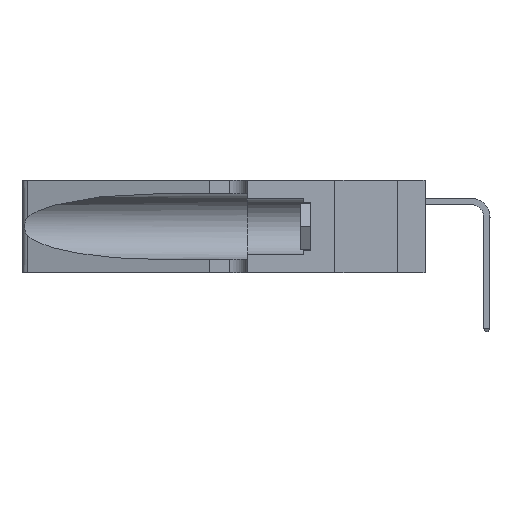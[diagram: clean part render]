
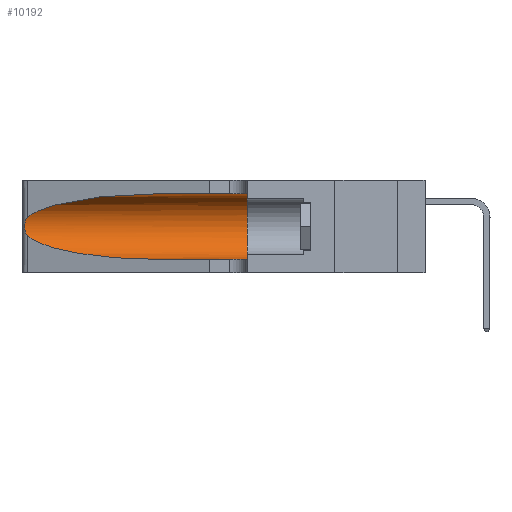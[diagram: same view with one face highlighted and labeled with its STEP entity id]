
A CAD part, left-side view. The second image highlights one B-rep face of the part: STEP entity #10192.
In plain terms, the highlighted cylindrical face has radius 3.308 mm (diameter 6.617 mm), a partial arc.
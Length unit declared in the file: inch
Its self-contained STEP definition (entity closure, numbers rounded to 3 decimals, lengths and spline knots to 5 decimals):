
#123 = CARTESIAN_POINT ( 'NONE',  ( 0.1305, 0.72297, 0.31525 ) ) ;
#985 = EDGE_LOOP ( 'NONE', ( #15493, #10895, #1255, #1177, #18945, #2947 ) ) ;
#1099 = FACE_OUTER_BOUND ( 'NONE', #985, .T. ) ;
#1177 = ORIENTED_EDGE ( 'NONE', *, *, #17334, .T. ) ;
#1226 = CARTESIAN_POINT ( 'NONE',  ( 0.1305, 0.35, 0.185 ) ) ;
#1255 = ORIENTED_EDGE ( 'NONE', *, *, #4249, .T. ) ;
#1370 = CARTESIAN_POINT ( 'NONE',  ( 0.26018, 1.23835, 0.19895 ) ) ;
#1497 = EDGE_CURVE ( 'NONE', #17183, #18191, #5691, .T. ) ;
#1720 = CARTESIAN_POINT ( 'NONE',  ( 0.25487, 1.22718, 0.22369 ) ) ;
#1990 = B_SPLINE_CURVE_WITH_KNOTS ( 'NONE', 3,
 ( #16617, #18098, #9055, #19607, #10561, #1370, #12128, #2957, #13651, #4505, #15153, #6045, #16682, #7584 ),
 .UNSPECIFIED., .F., .F.,
 ( 4, 2, 2, 2, 2, 2, 4 ),
 ( 0., 0.00027, 0.00053, 0.00107, 0.0016, 0.00187, 0.00214 ),
 .UNSPECIFIED. ) ;
#2947 = ORIENTED_EDGE ( 'NONE', *, *, #14438, .F. ) ;
#2957 = CARTESIAN_POINT ( 'NONE',  ( 0.26075, 1.23896, 0.178 ) ) ;
#3848 = VERTEX_POINT ( 'NONE', #16334 ) ;
#4218 =( BOUNDED_CURVE ( )  B_SPLINE_CURVE ( 3, ( #8485, #13027, #11481, #19059 ),
 .UNSPECIFIED., .F., .F. ) 
 B_SPLINE_CURVE_WITH_KNOTS ( ( 4, 4 ),
 ( 3.44316, 4.71239 ),
 .UNSPECIFIED. ) 
 CURVE ( )  GEOMETRIC_REPRESENTATION_ITEM ( )  RATIONAL_B_SPLINE_CURVE ( ( 1., 0.87, 0.87, 1. ) ) 
 REPRESENTATION_ITEM ( '' )  );
#4249 = EDGE_CURVE ( 'NONE', #9316, #14045, #4218, .T. ) ;
#4505 = CARTESIAN_POINT ( 'NONE',  ( 0.25856, 1.23593, 0.16098 ) ) ;
#4950 = VERTEX_POINT ( 'NONE', #123 ) ;
#5691 = CIRCLE ( 'NONE', #16948, 0.13025 ) ;
#6045 = CARTESIAN_POINT ( 'NONE',  ( 0.25639, 1.23186, 0.15144 ) ) ;
#6627 = DIRECTION ( 'NONE',  ( 0., 0., -1. ) ) ;
#6639 = EDGE_CURVE ( 'NONE', #3848, #9316, #1990, .T. ) ;
#6642 = LINE ( 'NONE', #9742, #11171 ) ;
#7527 = CARTESIAN_POINT ( 'NONE',  ( 0.25487, 1.22718, 0.14631 ) ) ;
#7531 = CARTESIAN_POINT ( 'NONE',  ( 0.1305, 0.35, 0.05475 ) ) ;
#7584 = CARTESIAN_POINT ( 'NONE',  ( 0.25487, 1.22718, 0.14631 ) ) ;
#7641 = EDGE_CURVE ( 'NONE', #4950, #3848, #11936, .T. ) ;
#7701 = DIRECTION ( 'NONE',  ( 0., -1., 0. ) ) ;
#8328 = CARTESIAN_POINT ( 'NONE',  ( 0.1305, 0.72297, 0.05475 ) ) ;
#8354 = CYLINDRICAL_SURFACE ( 'NONE', #16544, 0.13025 ) ;
#8446 = DIRECTION ( 'NONE',  ( 0., 0., 1. ) ) ;
#8485 = CARTESIAN_POINT ( 'NONE',  ( 0.25487, 1.22718, 0.14631 ) ) ;
#8526 = DIRECTION ( 'NONE',  ( 0., 1., 0. ) ) ;
#9055 = CARTESIAN_POINT ( 'NONE',  ( 0.25639, 1.23184, 0.21858 ) ) ;
#9316 = VERTEX_POINT ( 'NONE', #7527 ) ;
#9369 = CARTESIAN_POINT ( 'NONE',  ( 0.1305, 0.72297, 0.31525 ) ) ;
#9676 = DIRECTION ( 'NONE',  ( 0., -1., 0. ) ) ;
#9742 = CARTESIAN_POINT ( 'NONE',  ( 0.1305, 1.61858, 0.05475 ) ) ;
#10192 = ADVANCED_FACE ( 'NONE', ( #1099 ), #8354, .F. ) ;
#10561 = CARTESIAN_POINT ( 'NONE',  ( 0.25854, 1.2359, 0.20912 ) ) ;
#10895 = ORIENTED_EDGE ( 'NONE', *, *, #6639, .T. ) ;
#10909 = CARTESIAN_POINT ( 'NONE',  ( 0.2373, 1.15595, 0.28018 ) ) ;
#11171 = VECTOR ( 'NONE', #15811, 39.37008 ) ;
#11481 = CARTESIAN_POINT ( 'NONE',  ( 0.18966, 0.96281, 0.05475 ) ) ;
#11936 =( BOUNDED_CURVE ( )  B_SPLINE_CURVE ( 3, ( #9369, #16942, #10909, #1720 ),
 .UNSPECIFIED., .F., .F. ) 
 B_SPLINE_CURVE_WITH_KNOTS ( ( 4, 4 ),
 ( 1.5708, 2.84003 ),
 .UNSPECIFIED. ) 
 CURVE ( )  GEOMETRIC_REPRESENTATION_ITEM ( )  RATIONAL_B_SPLINE_CURVE ( ( 1., 0.87, 0.87, 1. ) ) 
 REPRESENTATION_ITEM ( '' )  );
#12128 = CARTESIAN_POINT ( 'NONE',  ( 0.26075, 1.23896, 0.19203 ) ) ;
#12750 = VECTOR ( 'NONE', #7701, 39.37008 ) ;
#13027 = CARTESIAN_POINT ( 'NONE',  ( 0.2373, 1.15595, 0.08982 ) ) ;
#13651 = CARTESIAN_POINT ( 'NONE',  ( 0.26017, 1.23833, 0.17102 ) ) ;
#14045 = VERTEX_POINT ( 'NONE', #8328 ) ;
#14194 = CARTESIAN_POINT ( 'NONE',  ( 0.1305, 1.61858, 0.185 ) ) ;
#14438 = EDGE_CURVE ( 'NONE', #4950, #17183, #19330, .T. ) ;
#15153 = CARTESIAN_POINT ( 'NONE',  ( 0.25789, 1.23486, 0.15765 ) ) ;
#15403 = CARTESIAN_POINT ( 'NONE',  ( 0.1305, 0.35, 0.31525 ) ) ;
#15493 = ORIENTED_EDGE ( 'NONE', *, *, #7641, .T. ) ;
#15811 = DIRECTION ( 'NONE',  ( 0., -1., 0. ) ) ;
#16334 = CARTESIAN_POINT ( 'NONE',  ( 0.25487, 1.22718, 0.22369 ) ) ;
#16544 = AXIS2_PLACEMENT_3D ( 'NONE', #14194, #9676, #6627 ) ;
#16617 = CARTESIAN_POINT ( 'NONE',  ( 0.25487, 1.22718, 0.22369 ) ) ;
#16682 = CARTESIAN_POINT ( 'NONE',  ( 0.25555, 1.22993, 0.14849 ) ) ;
#16942 = CARTESIAN_POINT ( 'NONE',  ( 0.18966, 0.96281, 0.31525 ) ) ;
#16948 = AXIS2_PLACEMENT_3D ( 'NONE', #1226, #8526, #8446 ) ;
#17183 = VERTEX_POINT ( 'NONE', #15403 ) ;
#17334 = EDGE_CURVE ( 'NONE', #14045, #18191, #6642, .T. ) ;
#18098 = CARTESIAN_POINT ( 'NONE',  ( 0.25555, 1.22994, 0.2215 ) ) ;
#18191 = VERTEX_POINT ( 'NONE', #7531 ) ;
#18271 = CARTESIAN_POINT ( 'NONE',  ( 0.1305, 1.61858, 0.31525 ) ) ;
#18945 = ORIENTED_EDGE ( 'NONE', *, *, #1497, .F. ) ;
#19059 = CARTESIAN_POINT ( 'NONE',  ( 0.1305, 0.72297, 0.05475 ) ) ;
#19330 = LINE ( 'NONE', #18271, #12750 ) ;
#19607 = CARTESIAN_POINT ( 'NONE',  ( 0.25787, 1.23484, 0.2124 ) ) ;
